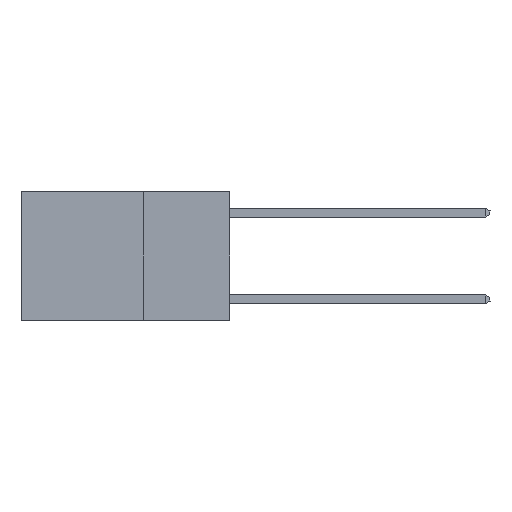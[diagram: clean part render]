
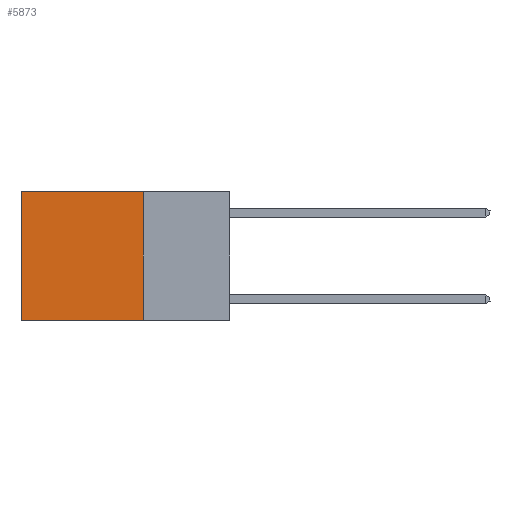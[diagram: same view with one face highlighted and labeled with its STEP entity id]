
A CAD part, left-side view. The second image highlights one B-rep face of the part: STEP entity #5873.
In plain terms, the highlighted planar face has unit normal (-1, 0, 0).
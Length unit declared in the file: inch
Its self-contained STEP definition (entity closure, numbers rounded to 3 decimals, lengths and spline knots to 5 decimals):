
#272 = DIRECTION ( 'NONE',  ( 0., 1., 0. ) ) ;
#1432 = VERTEX_POINT ( 'NONE', #19289 ) ;
#2566 = FACE_OUTER_BOUND ( 'NONE', #14545, .T. ) ;
#3608 = LINE ( 'NONE', #17615, #19083 ) ;
#5873 = ADVANCED_FACE ( 'NONE', ( #2566 ), #20708, .F. ) ;
#6742 = ORIENTED_EDGE ( 'NONE', *, *, #28064, .F. ) ;
#7553 = VECTOR ( 'NONE', #272, 39.37008 ) ;
#8484 = VECTOR ( 'NONE', #22705, 39.37008 ) ;
#8768 = DIRECTION ( 'NONE',  ( 1., 0., 0. ) ) ;
#9293 = EDGE_CURVE ( 'NONE', #20370, #20253, #13425, .T. ) ;
#11043 = CARTESIAN_POINT ( 'NONE',  ( 0.2625, 0.6, 0. ) ) ;
#11599 = CARTESIAN_POINT ( 'NONE',  ( 0.2625, 0.6, 0. ) ) ;
#13425 = LINE ( 'NONE', #15801, #7553 ) ;
#13561 = DIRECTION ( 'NONE',  ( 0., 0., -1. ) ) ;
#13628 = EDGE_CURVE ( 'NONE', #20253, #1432, #20255, .T. ) ;
#13629 = LINE ( 'NONE', #27350, #8484 ) ;
#14545 = EDGE_LOOP ( 'NONE', ( #14799, #21958, #6742, #29258 ) ) ;
#14799 = ORIENTED_EDGE ( 'NONE', *, *, #13628, .T. ) ;
#15801 = CARTESIAN_POINT ( 'NONE',  ( 0.2625, 0.25, 0. ) ) ;
#16251 = CARTESIAN_POINT ( 'NONE',  ( 0.2625, 0.25, 0. ) ) ;
#17150 = VERTEX_POINT ( 'NONE', #20438 ) ;
#17615 = CARTESIAN_POINT ( 'NONE',  ( 0.2625, 0.25, -0.37 ) ) ;
#18449 = DIRECTION ( 'NONE',  ( 0., 0., -1. ) ) ;
#19083 = VECTOR ( 'NONE', #28791, 39.37008 ) ;
#19289 = CARTESIAN_POINT ( 'NONE',  ( 0.2625, 0.6, -0.37 ) ) ;
#20253 = VERTEX_POINT ( 'NONE', #11043 ) ;
#20255 = LINE ( 'NONE', #11599, #20893 ) ;
#20370 = VERTEX_POINT ( 'NONE', #29353 ) ;
#20438 = CARTESIAN_POINT ( 'NONE',  ( 0.2625, 0.25, -0.37 ) ) ;
#20708 = PLANE ( 'NONE',  #27952 ) ;
#20893 = VECTOR ( 'NONE', #18449, 39.37008 ) ;
#21003 = EDGE_CURVE ( 'NONE', #17150, #1432, #3608, .T. ) ;
#21958 = ORIENTED_EDGE ( 'NONE', *, *, #21003, .F. ) ;
#22705 = DIRECTION ( 'NONE',  ( 0., 0., -1. ) ) ;
#27350 = CARTESIAN_POINT ( 'NONE',  ( 0.2625, 0.25, 0. ) ) ;
#27952 = AXIS2_PLACEMENT_3D ( 'NONE', #16251, #8768, #13561 ) ;
#28064 = EDGE_CURVE ( 'NONE', #20370, #17150, #13629, .T. ) ;
#28791 = DIRECTION ( 'NONE',  ( 0., 1., 0. ) ) ;
#29258 = ORIENTED_EDGE ( 'NONE', *, *, #9293, .T. ) ;
#29353 = CARTESIAN_POINT ( 'NONE',  ( 0.2625, 0.25, 0. ) ) ;
